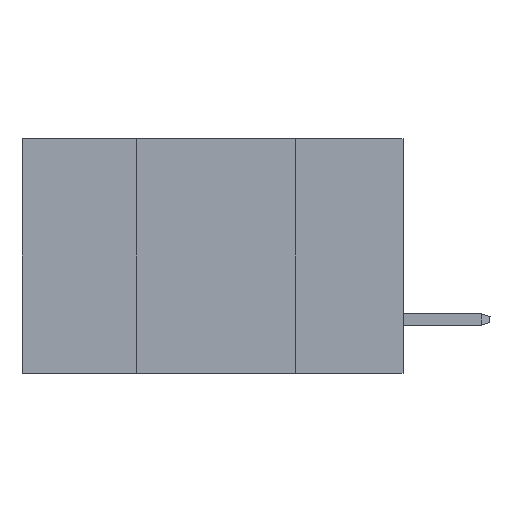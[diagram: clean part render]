
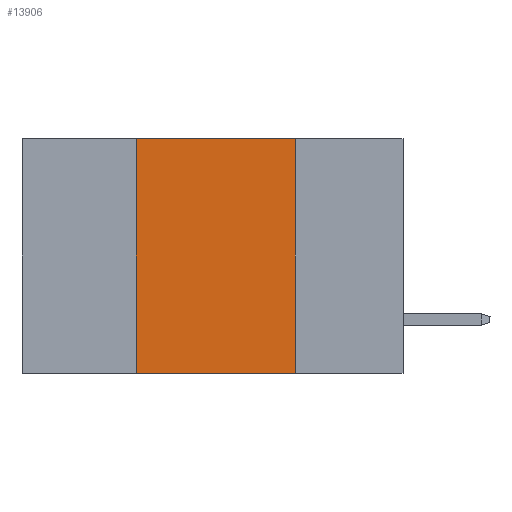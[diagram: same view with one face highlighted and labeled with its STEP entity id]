
A CAD part, left-side view. The second image highlights one B-rep face of the part: STEP entity #13906.
In plain terms, the highlighted planar face has unit normal (-1, 0, 0).
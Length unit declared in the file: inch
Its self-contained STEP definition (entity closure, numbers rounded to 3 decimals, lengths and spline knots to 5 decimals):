
#454 = ORIENTED_EDGE ( 'NONE', *, *, #32605, .T. ) ;
#728 = VERTEX_POINT ( 'NONE', #4035 ) ;
#865 = ORIENTED_EDGE ( 'NONE', *, *, #23874, .F. ) ;
#2325 = CARTESIAN_POINT ( 'NONE',  ( 0., 0.17, -0.37 ) ) ;
#2553 = LINE ( 'NONE', #13840, #27046 ) ;
#4035 = CARTESIAN_POINT ( 'NONE',  ( 0., 0.42, 0. ) ) ;
#5299 = DIRECTION ( 'NONE',  ( 0., -1., 0. ) ) ;
#7515 = VERTEX_POINT ( 'NONE', #30690 ) ;
#8873 = VERTEX_POINT ( 'NONE', #21918 ) ;
#9375 = CARTESIAN_POINT ( 'NONE',  ( 0., 0.42, 0. ) ) ;
#12385 = LINE ( 'NONE', #9375, #27915 ) ;
#12807 = DIRECTION ( 'NONE',  ( 0., 0., -1. ) ) ;
#13840 = CARTESIAN_POINT ( 'NONE',  ( 0., 0.17, 0. ) ) ;
#13906 = ADVANCED_FACE ( 'NONE', ( #18421 ), #15795, .F. ) ;
#14016 = AXIS2_PLACEMENT_3D ( 'NONE', #17911, #26558, #12807 ) ;
#15795 = PLANE ( 'NONE',  #14016 ) ;
#17159 = EDGE_CURVE ( 'NONE', #728, #8873, #18691, .T. ) ;
#17586 = CARTESIAN_POINT ( 'NONE',  ( 0., 0.6, -0.37 ) ) ;
#17911 = CARTESIAN_POINT ( 'NONE',  ( 0., 0.6, 0. ) ) ;
#18421 = FACE_OUTER_BOUND ( 'NONE', #26982, .T. ) ;
#18691 = LINE ( 'NONE', #29491, #24308 ) ;
#18807 = ORIENTED_EDGE ( 'NONE', *, *, #23228, .F. ) ;
#19300 = ORIENTED_EDGE ( 'NONE', *, *, #17159, .F. ) ;
#21918 = CARTESIAN_POINT ( 'NONE',  ( 0., 0.17, 0. ) ) ;
#23228 = EDGE_CURVE ( 'NONE', #8873, #30988, #2553, .T. ) ;
#23874 = EDGE_CURVE ( 'NONE', #7515, #728, #12385, .T. ) ;
#24308 = VECTOR ( 'NONE', #5299, 39.37008 ) ;
#25613 = DIRECTION ( 'NONE',  ( 0., 0., 1. ) ) ;
#26229 = DIRECTION ( 'NONE',  ( 0., -1., 0. ) ) ;
#26558 = DIRECTION ( 'NONE',  ( 1., 0., 0. ) ) ;
#26982 = EDGE_LOOP ( 'NONE', ( #18807, #19300, #865, #454 ) ) ;
#27046 = VECTOR ( 'NONE', #33608, 39.37008 ) ;
#27915 = VECTOR ( 'NONE', #25613, 39.37008 ) ;
#28609 = VECTOR ( 'NONE', #26229, 39.37008 ) ;
#29491 = CARTESIAN_POINT ( 'NONE',  ( 0., 0.6, 0. ) ) ;
#30690 = CARTESIAN_POINT ( 'NONE',  ( 0., 0.42, -0.37 ) ) ;
#30988 = VERTEX_POINT ( 'NONE', #2325 ) ;
#31055 = LINE ( 'NONE', #17586, #28609 ) ;
#32605 = EDGE_CURVE ( 'NONE', #7515, #30988, #31055, .T. ) ;
#33608 = DIRECTION ( 'NONE',  ( 0., 0., -1. ) ) ;
